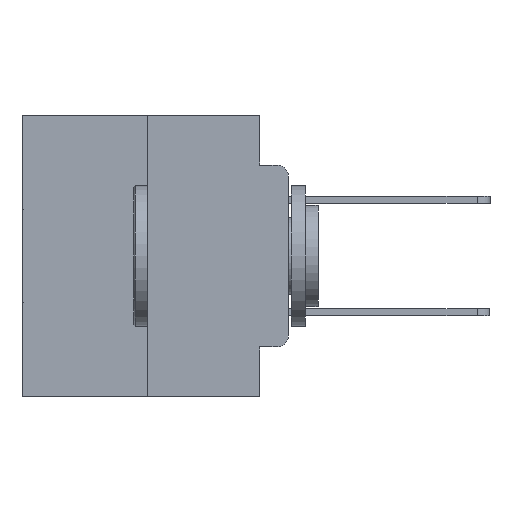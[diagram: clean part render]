
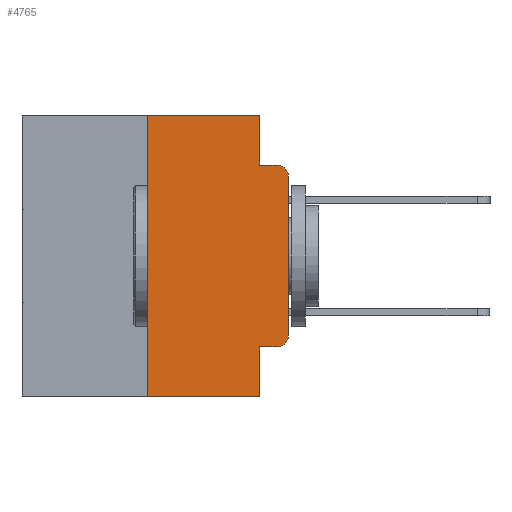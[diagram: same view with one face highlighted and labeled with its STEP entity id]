
A CAD part, left-side view. The second image highlights one B-rep face of the part: STEP entity #4765.
In plain terms, the highlighted planar face has unit normal (-1, 0, 0).
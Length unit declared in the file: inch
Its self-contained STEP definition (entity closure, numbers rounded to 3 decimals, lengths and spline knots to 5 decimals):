
#16 = DIRECTION ( 'NONE',  ( 0., 0., 1. ) ) ;
#795 = VECTOR ( 'NONE', #25907, 39.37008 ) ;
#1227 = LINE ( 'NONE', #24768, #5163 ) ;
#1445 = ORIENTED_EDGE ( 'NONE', *, *, #4493, .F. ) ;
#1474 = ORIENTED_EDGE ( 'NONE', *, *, #7911, .F. ) ;
#1607 = ORIENTED_EDGE ( 'NONE', *, *, #24214, .T. ) ;
#1852 = EDGE_CURVE ( 'NONE', #11712, #18120, #3601, .T. ) ;
#2352 = LINE ( 'NONE', #15636, #13645 ) ;
#2985 = LINE ( 'NONE', #12799, #795 ) ;
#3351 = ORIENTED_EDGE ( 'NONE', *, *, #21317, .F. ) ;
#3601 = LINE ( 'NONE', #12712, #10296 ) ;
#4339 = VECTOR ( 'NONE', #10520, 39.37008 ) ;
#4493 = EDGE_CURVE ( 'NONE', #18120, #5926, #2352, .T. ) ;
#4765 = ADVANCED_FACE ( 'NONE', ( #7275 ), #5480, .F. ) ;
#4776 = ORIENTED_EDGE ( 'NONE', *, *, #16935, .T. ) ;
#4908 = ORIENTED_EDGE ( 'NONE', *, *, #15475, .F. ) ;
#5163 = VECTOR ( 'NONE', #13982, 39.37008 ) ;
#5480 = PLANE ( 'NONE',  #24016 ) ;
#5926 = VERTEX_POINT ( 'NONE', #24777 ) ;
#6062 = VERTEX_POINT ( 'NONE', #16602 ) ;
#6182 = DIRECTION ( 'NONE',  ( 0., -1., 0. ) ) ;
#6939 = DIRECTION ( 'NONE',  ( 0., -1., 0. ) ) ;
#6968 = EDGE_CURVE ( 'NONE', #26779, #13478, #9268, .T. ) ;
#7275 = FACE_OUTER_BOUND ( 'NONE', #16656, .T. ) ;
#7358 = ORIENTED_EDGE ( 'NONE', *, *, #21847, .T. ) ;
#7703 = ORIENTED_EDGE ( 'NONE', *, *, #6968, .T. ) ;
#7735 = DIRECTION ( 'NONE',  ( 1., 0., 0. ) ) ;
#7751 = AXIS2_PLACEMENT_3D ( 'NONE', #24440, #11275, #26641 ) ;
#7911 = EDGE_CURVE ( 'NONE', #20878, #6062, #16967, .T. ) ;
#9266 = CARTESIAN_POINT ( 'NONE',  ( 0., 0.25, -0.5 ) ) ;
#9268 = CIRCLE ( 'NONE', #7751, 0.02 ) ;
#10296 = VECTOR ( 'NONE', #25819, 39.37008 ) ;
#10520 = DIRECTION ( 'NONE',  ( 0., 0., -1. ) ) ;
#11275 = DIRECTION ( 'NONE',  ( -1., 0., 0. ) ) ;
#11644 = CARTESIAN_POINT ( 'NONE',  ( 0., 0.02, -0.1085 ) ) ;
#11682 = LINE ( 'NONE', #17349, #16906 ) ;
#11712 = VERTEX_POINT ( 'NONE', #9266 ) ;
#12405 = ORIENTED_EDGE ( 'NONE', *, *, #1852, .F. ) ;
#12496 = ORIENTED_EDGE ( 'NONE', *, *, #24589, .T. ) ;
#12712 = CARTESIAN_POINT ( 'NONE',  ( 0., 0.25, 0. ) ) ;
#12799 = CARTESIAN_POINT ( 'NONE',  ( 0., 0.051, -0.0885 ) ) ;
#12836 = VERTEX_POINT ( 'NONE', #15319 ) ;
#13471 = DIRECTION ( 'NONE',  ( 0., -1., 0. ) ) ;
#13478 = VERTEX_POINT ( 'NONE', #25625 ) ;
#13645 = VECTOR ( 'NONE', #13471, 39.37008 ) ;
#13902 = DIRECTION ( 'NONE',  ( 0., 0., -1. ) ) ;
#13982 = DIRECTION ( 'NONE',  ( 0., 0., -1. ) ) ;
#15319 = CARTESIAN_POINT ( 'NONE',  ( 0., 0.051, -0.0885 ) ) ;
#15475 = EDGE_CURVE ( 'NONE', #12836, #28655, #2985, .T. ) ;
#15616 = CARTESIAN_POINT ( 'NONE',  ( 0., 0.02, -0.4115 ) ) ;
#15636 = CARTESIAN_POINT ( 'NONE',  ( 0., 0.473, 0. ) ) ;
#15671 = VECTOR ( 'NONE', #6939, 39.37008 ) ;
#16602 = CARTESIAN_POINT ( 'NONE',  ( 0., 0.051, -0.5 ) ) ;
#16656 = EDGE_LOOP ( 'NONE', ( #4776, #1607, #4908, #3351, #1445, #12405, #12496, #1474, #7358, #7703 ) ) ;
#16906 = VECTOR ( 'NONE', #6182, 39.37008 ) ;
#16935 = EDGE_CURVE ( 'NONE', #13478, #17907, #18053, .T. ) ;
#16967 = LINE ( 'NONE', #25900, #4339 ) ;
#17308 = CARTESIAN_POINT ( 'NONE',  ( 0., 0., -0.1085 ) ) ;
#17349 = CARTESIAN_POINT ( 'NONE',  ( 0., 0.473, -0.5 ) ) ;
#17907 = VERTEX_POINT ( 'NONE', #17308 ) ;
#18053 = LINE ( 'NONE', #24499, #28262 ) ;
#18120 = VERTEX_POINT ( 'NONE', #26722 ) ;
#20227 = AXIS2_PLACEMENT_3D ( 'NONE', #11644, #26991, #13902 ) ;
#20878 = VERTEX_POINT ( 'NONE', #25549 ) ;
#21053 = CARTESIAN_POINT ( 'NONE',  ( 0., 0.473, 0. ) ) ;
#21317 = EDGE_CURVE ( 'NONE', #5926, #12836, #1227, .T. ) ;
#21847 = EDGE_CURVE ( 'NONE', #20878, #26779, #27250, .T. ) ;
#22036 = CIRCLE ( 'NONE', #20227, 0.02 ) ;
#23236 = DIRECTION ( 'NONE',  ( 0., 0., -1. ) ) ;
#23616 = CARTESIAN_POINT ( 'NONE',  ( 0., 0.02, -0.0885 ) ) ;
#24016 = AXIS2_PLACEMENT_3D ( 'NONE', #21053, #7735, #23236 ) ;
#24214 = EDGE_CURVE ( 'NONE', #17907, #28655, #22036, .T. ) ;
#24440 = CARTESIAN_POINT ( 'NONE',  ( 0., 0.02, -0.3915 ) ) ;
#24499 = CARTESIAN_POINT ( 'NONE',  ( 0., 0., 0. ) ) ;
#24544 = CARTESIAN_POINT ( 'NONE',  ( 0., 0.051, -0.4115 ) ) ;
#24589 = EDGE_CURVE ( 'NONE', #11712, #6062, #11682, .T. ) ;
#24768 = CARTESIAN_POINT ( 'NONE',  ( 0., 0.051, 0. ) ) ;
#24777 = CARTESIAN_POINT ( 'NONE',  ( 0., 0.051, 0. ) ) ;
#25549 = CARTESIAN_POINT ( 'NONE',  ( 0., 0.051, -0.4115 ) ) ;
#25625 = CARTESIAN_POINT ( 'NONE',  ( 0., 0., -0.3915 ) ) ;
#25819 = DIRECTION ( 'NONE',  ( 0., 0., 1. ) ) ;
#25900 = CARTESIAN_POINT ( 'NONE',  ( 0., 0.051, 0. ) ) ;
#25907 = DIRECTION ( 'NONE',  ( 0., -1., 0. ) ) ;
#26641 = DIRECTION ( 'NONE',  ( 0., 0., -1. ) ) ;
#26722 = CARTESIAN_POINT ( 'NONE',  ( 0., 0.25, 0. ) ) ;
#26779 = VERTEX_POINT ( 'NONE', #15616 ) ;
#26991 = DIRECTION ( 'NONE',  ( -1., 0., 0. ) ) ;
#27250 = LINE ( 'NONE', #24544, #15671 ) ;
#28262 = VECTOR ( 'NONE', #16, 39.37008 ) ;
#28655 = VERTEX_POINT ( 'NONE', #23616 ) ;
